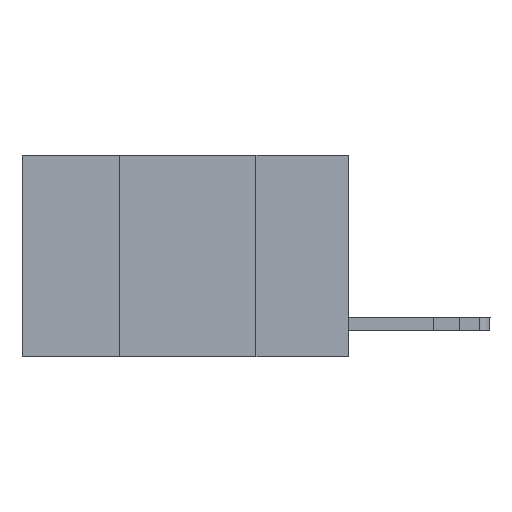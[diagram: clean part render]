
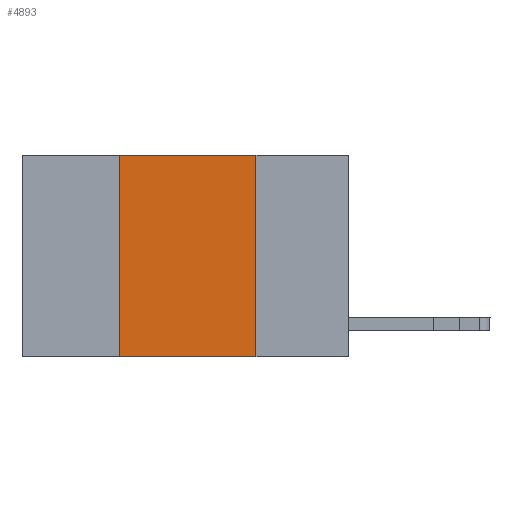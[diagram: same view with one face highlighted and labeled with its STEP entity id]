
A CAD part, left-side view. The second image highlights one B-rep face of the part: STEP entity #4893.
In plain terms, the highlighted planar face has unit normal (-1, 0, 0).
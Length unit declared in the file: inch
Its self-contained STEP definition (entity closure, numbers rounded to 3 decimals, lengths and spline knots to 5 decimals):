
#374 = CARTESIAN_POINT ( 'NONE',  ( 0., 0.42, -0.37 ) ) ;
#1569 = VERTEX_POINT ( 'NONE', #374 ) ;
#2326 = CARTESIAN_POINT ( 'NONE',  ( 0., 0.17, -0.37 ) ) ;
#2466 = EDGE_CURVE ( 'NONE', #1569, #21383, #6810, .T. ) ;
#2477 = PLANE ( 'NONE',  #8985 ) ;
#2497 = CARTESIAN_POINT ( 'NONE',  ( 0., 0.42, 0. ) ) ;
#2553 = EDGE_LOOP ( 'NONE', ( #19727, #7017, #11655, #8115 ) ) ;
#2775 = DIRECTION ( 'NONE',  ( 0., -1., 0. ) ) ;
#4848 = VERTEX_POINT ( 'NONE', #2326 ) ;
#4893 = ADVANCED_FACE ( 'NONE', ( #12143 ), #2477, .F. ) ;
#5103 = DIRECTION ( 'NONE',  ( 0., 0., -1. ) ) ;
#5515 = EDGE_CURVE ( 'NONE', #1569, #4848, #21283, .T. ) ;
#5671 = CARTESIAN_POINT ( 'NONE',  ( 0., 0.17, 0. ) ) ;
#6008 = DIRECTION ( 'NONE',  ( 0., 0., -1. ) ) ;
#6810 = LINE ( 'NONE', #2497, #19532 ) ;
#7017 = ORIENTED_EDGE ( 'NONE', *, *, #12904, .F. ) ;
#7523 = VECTOR ( 'NONE', #13023, 39.37008 ) ;
#8115 = ORIENTED_EDGE ( 'NONE', *, *, #5515, .T. ) ;
#8152 = LINE ( 'NONE', #21784, #16839 ) ;
#8985 = AXIS2_PLACEMENT_3D ( 'NONE', #14682, #16402, #6008 ) ;
#9441 = CARTESIAN_POINT ( 'NONE',  ( 0., 0.6, -0.37 ) ) ;
#10671 = CARTESIAN_POINT ( 'NONE',  ( 0., 0.42, 0. ) ) ;
#11655 = ORIENTED_EDGE ( 'NONE', *, *, #2466, .F. ) ;
#12054 = CARTESIAN_POINT ( 'NONE',  ( 0., 0.17, 0. ) ) ;
#12143 = FACE_OUTER_BOUND ( 'NONE', #2553, .T. ) ;
#12904 = EDGE_CURVE ( 'NONE', #21383, #13379, #8152, .T. ) ;
#13023 = DIRECTION ( 'NONE',  ( 0., -1., 0. ) ) ;
#13379 = VERTEX_POINT ( 'NONE', #5671 ) ;
#13748 = EDGE_CURVE ( 'NONE', #13379, #4848, #17870, .T. ) ;
#14682 = CARTESIAN_POINT ( 'NONE',  ( 0., 0.6, 0. ) ) ;
#16402 = DIRECTION ( 'NONE',  ( 1., 0., 0. ) ) ;
#16433 = DIRECTION ( 'NONE',  ( 0., 0., 1. ) ) ;
#16839 = VECTOR ( 'NONE', #2775, 39.37008 ) ;
#17870 = LINE ( 'NONE', #12054, #21876 ) ;
#19532 = VECTOR ( 'NONE', #16433, 39.37008 ) ;
#19727 = ORIENTED_EDGE ( 'NONE', *, *, #13748, .F. ) ;
#21283 = LINE ( 'NONE', #9441, #7523 ) ;
#21383 = VERTEX_POINT ( 'NONE', #10671 ) ;
#21784 = CARTESIAN_POINT ( 'NONE',  ( 0., 0.6, 0. ) ) ;
#21876 = VECTOR ( 'NONE', #5103, 39.37008 ) ;
